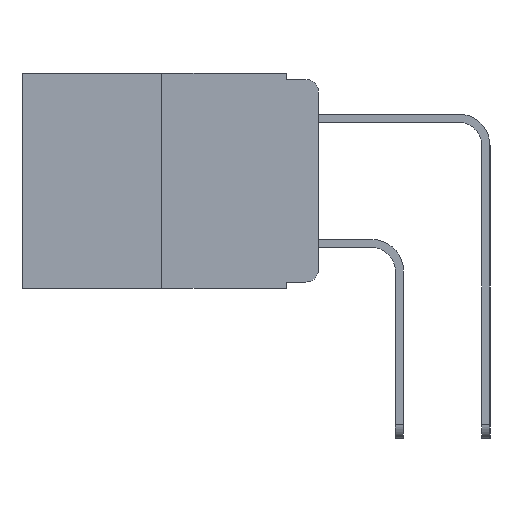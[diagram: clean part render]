
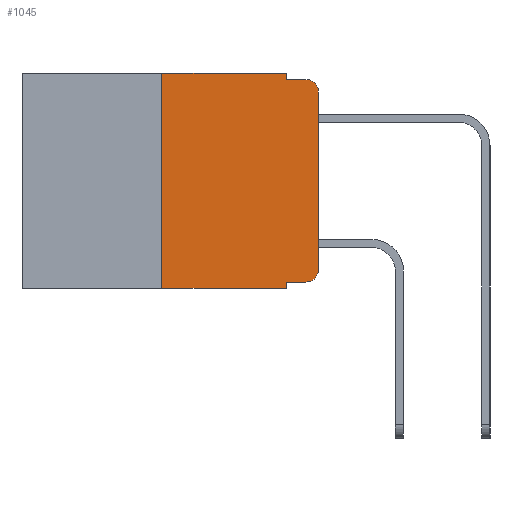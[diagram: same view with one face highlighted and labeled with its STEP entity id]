
A CAD part, left-side view. The second image highlights one B-rep face of the part: STEP entity #1045.
In plain terms, the highlighted planar face has unit normal (-1, 0, 0).
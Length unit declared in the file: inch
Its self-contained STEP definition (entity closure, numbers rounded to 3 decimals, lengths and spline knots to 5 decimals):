
#10 = CARTESIAN_POINT ( 'NONE',  ( 0., 0.051, -0.333 ) ) ;
#353 = EDGE_CURVE ( 'NONE', #9995, #1051, #13641, .T. ) ;
#904 = DIRECTION ( 'NONE',  ( 0., 0., 1. ) ) ;
#1045 = ADVANCED_FACE ( 'NONE', ( #7937 ), #10830, .F. ) ;
#1051 = VERTEX_POINT ( 'NONE', #7826 ) ;
#1203 = LINE ( 'NONE', #9462, #10513 ) ;
#1295 = DIRECTION ( 'NONE',  ( 0., -1., 0. ) ) ;
#1562 = CARTESIAN_POINT ( 'NONE',  ( 0., 0.051, -0.333 ) ) ;
#2181 = CARTESIAN_POINT ( 'NONE',  ( 0., 0.051, 0. ) ) ;
#2592 = EDGE_CURVE ( 'NONE', #5189, #4219, #7913, .T. ) ;
#2807 = VERTEX_POINT ( 'NONE', #7591 ) ;
#3045 = DIRECTION ( 'NONE',  ( 0., 0., -1. ) ) ;
#3255 = DIRECTION ( 'NONE',  ( 0., -1., 0. ) ) ;
#3275 = CARTESIAN_POINT ( 'NONE',  ( 0., 0.051, -0.01 ) ) ;
#3455 = DIRECTION ( 'NONE',  ( 0., 0., -1. ) ) ;
#3534 = ORIENTED_EDGE ( 'NONE', *, *, #2592, .F. ) ;
#3732 = VECTOR ( 'NONE', #3045, 39.37008 ) ;
#4219 = VERTEX_POINT ( 'NONE', #7157 ) ;
#4309 = ORIENTED_EDGE ( 'NONE', *, *, #10897, .F. ) ;
#4318 = CARTESIAN_POINT ( 'NONE',  ( 0., 0., 0. ) ) ;
#4501 = VECTOR ( 'NONE', #1295, 39.37008 ) ;
#4651 = VECTOR ( 'NONE', #3255, 39.37008 ) ;
#4691 = ORIENTED_EDGE ( 'NONE', *, *, #353, .T. ) ;
#4788 = EDGE_CURVE ( 'NONE', #2807, #9037, #13903, .T. ) ;
#5189 = VERTEX_POINT ( 'NONE', #14115 ) ;
#5293 = DIRECTION ( 'NONE',  ( -1., 0., 0. ) ) ;
#5486 = CARTESIAN_POINT ( 'NONE',  ( 0., 0.051, 0. ) ) ;
#5492 = ORIENTED_EDGE ( 'NONE', *, *, #8865, .T. ) ;
#5572 = DIRECTION ( 'NONE',  ( 0., 0., 1. ) ) ;
#6347 = CARTESIAN_POINT ( 'NONE',  ( 0., 0.02, -0.313 ) ) ;
#6744 = EDGE_CURVE ( 'NONE', #9464, #4219, #9305, .T. ) ;
#7157 = CARTESIAN_POINT ( 'NONE',  ( 0., 0.02, -0.01 ) ) ;
#7176 = ORIENTED_EDGE ( 'NONE', *, *, #7300, .F. ) ;
#7300 = EDGE_CURVE ( 'NONE', #13199, #13968, #8745, .T. ) ;
#7329 = EDGE_LOOP ( 'NONE', ( #15375, #12720, #3534, #9963, #7176, #4309, #4691, #8335, #5492, #8705 ) ) ;
#7572 = DIRECTION ( 'NONE',  ( 0., 0., -1. ) ) ;
#7591 = CARTESIAN_POINT ( 'NONE',  ( 0., 0.02, -0.333 ) ) ;
#7826 = CARTESIAN_POINT ( 'NONE',  ( 0., 0.051, -0.343 ) ) ;
#7913 = LINE ( 'NONE', #3275, #4651 ) ;
#7937 = FACE_OUTER_BOUND ( 'NONE', #7329, .T. ) ;
#8335 = ORIENTED_EDGE ( 'NONE', *, *, #9376, .F. ) ;
#8499 = LINE ( 'NONE', #10, #4501 ) ;
#8506 = EDGE_CURVE ( 'NONE', #13968, #5189, #10140, .T. ) ;
#8705 = ORIENTED_EDGE ( 'NONE', *, *, #4788, .T. ) ;
#8745 = LINE ( 'NONE', #11194, #14184 ) ;
#8865 = EDGE_CURVE ( 'NONE', #11919, #2807, #8499, .T. ) ;
#9037 = VERTEX_POINT ( 'NONE', #13591 ) ;
#9144 = AXIS2_PLACEMENT_3D ( 'NONE', #6347, #14562, #7572 ) ;
#9305 = CIRCLE ( 'NONE', #9648, 0.02 ) ;
#9376 = EDGE_CURVE ( 'NONE', #11919, #1051, #13602, .T. ) ;
#9462 = CARTESIAN_POINT ( 'NONE',  ( 0., 0.25, 0. ) ) ;
#9464 = VERTEX_POINT ( 'NONE', #13172 ) ;
#9648 = AXIS2_PLACEMENT_3D ( 'NONE', #12409, #5293, #13583 ) ;
#9963 = ORIENTED_EDGE ( 'NONE', *, *, #8506, .F. ) ;
#9995 = VERTEX_POINT ( 'NONE', #10931 ) ;
#10140 = LINE ( 'NONE', #5486, #3732 ) ;
#10235 = CARTESIAN_POINT ( 'NONE',  ( 0., 0.25, 0. ) ) ;
#10513 = VECTOR ( 'NONE', #904, 39.37008 ) ;
#10830 = PLANE ( 'NONE',  #13320 ) ;
#10897 = EDGE_CURVE ( 'NONE', #9995, #13199, #1203, .T. ) ;
#10931 = CARTESIAN_POINT ( 'NONE',  ( 0., 0.25, -0.343 ) ) ;
#11194 = CARTESIAN_POINT ( 'NONE',  ( 0., 0.473, 0. ) ) ;
#11547 = DIRECTION ( 'NONE',  ( 0., 0., -1. ) ) ;
#11919 = VERTEX_POINT ( 'NONE', #1562 ) ;
#12394 = DIRECTION ( 'NONE',  ( 0., -1., 0. ) ) ;
#12409 = CARTESIAN_POINT ( 'NONE',  ( 0., 0.02, -0.03 ) ) ;
#12443 = LINE ( 'NONE', #4318, #14407 ) ;
#12720 = ORIENTED_EDGE ( 'NONE', *, *, #6744, .T. ) ;
#13172 = CARTESIAN_POINT ( 'NONE',  ( 0., 0., -0.03 ) ) ;
#13199 = VERTEX_POINT ( 'NONE', #10235 ) ;
#13235 = VECTOR ( 'NONE', #3455, 39.37008 ) ;
#13270 = VECTOR ( 'NONE', #13859, 39.37008 ) ;
#13320 = AXIS2_PLACEMENT_3D ( 'NONE', #14682, #13423, #11547 ) ;
#13423 = DIRECTION ( 'NONE',  ( 1., 0., 0. ) ) ;
#13583 = DIRECTION ( 'NONE',  ( 0., 0., -1. ) ) ;
#13591 = CARTESIAN_POINT ( 'NONE',  ( 0., 0., -0.313 ) ) ;
#13602 = LINE ( 'NONE', #2181, #13235 ) ;
#13641 = LINE ( 'NONE', #14745, #13270 ) ;
#13859 = DIRECTION ( 'NONE',  ( 0., -1., 0. ) ) ;
#13903 = CIRCLE ( 'NONE', #9144, 0.02 ) ;
#13968 = VERTEX_POINT ( 'NONE', #14771 ) ;
#14052 = EDGE_CURVE ( 'NONE', #9037, #9464, #12443, .T. ) ;
#14115 = CARTESIAN_POINT ( 'NONE',  ( 0., 0.051, -0.01 ) ) ;
#14184 = VECTOR ( 'NONE', #12394, 39.37008 ) ;
#14407 = VECTOR ( 'NONE', #5572, 39.37008 ) ;
#14562 = DIRECTION ( 'NONE',  ( -1., 0., 0. ) ) ;
#14682 = CARTESIAN_POINT ( 'NONE',  ( 0., 0.473, 0. ) ) ;
#14745 = CARTESIAN_POINT ( 'NONE',  ( 0., 0.473, -0.343 ) ) ;
#14771 = CARTESIAN_POINT ( 'NONE',  ( 0., 0.051, 0. ) ) ;
#15375 = ORIENTED_EDGE ( 'NONE', *, *, #14052, .T. ) ;
